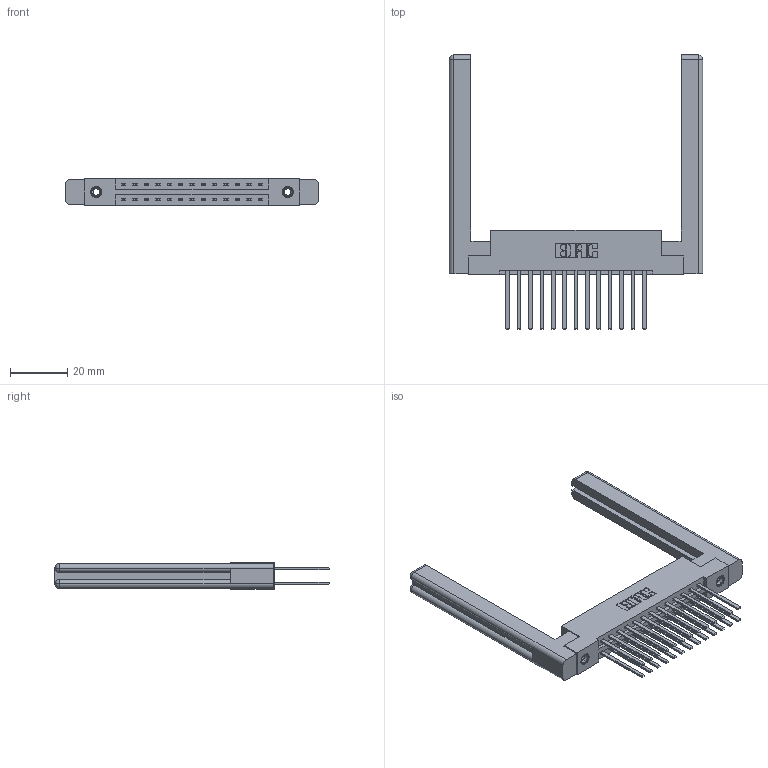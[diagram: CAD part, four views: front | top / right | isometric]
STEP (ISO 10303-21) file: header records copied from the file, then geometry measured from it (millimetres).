
FILE_DESCRIPTION (( 'STEP AP203' ), '1' );
FILE_NAME ('387-026-544-258.STEP', '2019-10-16T20:25:09', ( '' ), ( '' ), 'SwSTEP 2.0', 'SolidWorks 2016', '' );
FILE_SCHEMA (( 'CONFIG_CONTROL_DESIGN' ));
Length unit declared in the file: inch
Products named in the file (5): 387-026-544-258; 337 Part_Flush Mounting Lugs - 0.156 Dia-TI; 345-292-001_345-293-144; 345-250-001_345-250-001-102; 307-220-058
Assembly tree (31 placements, depth 2):
  387-026-544-258
    337 Part_Flush Mounting Lugs - 0.156 Dia-TI
    345-292-001_345-293-144  x26
    345-250-001_345-250-001-102  x2
    307-220-058  x2
Bounding box: 88.14 x 95.38 x 9.4 mm (x, y, z)
Volume: 16409.5 mm3; surface area: 16432.2 mm2
Topology: 31 solids, 31 shells, 1504 faces, 4383 edges, 2874 vertices
Faces by surface type: plane 1038, cylinder 442, cone 12, torus 12
Entity records: 16280 total; most frequent: CARTESIAN_POINT 2773, ORIENTED_EDGE 2648, DIRECTION 2424, EDGE_CURVE 1324, LINE 1152, VECTOR 1152, VERTEX_POINT 874, AXIS2_PLACEMENT_3D 636
